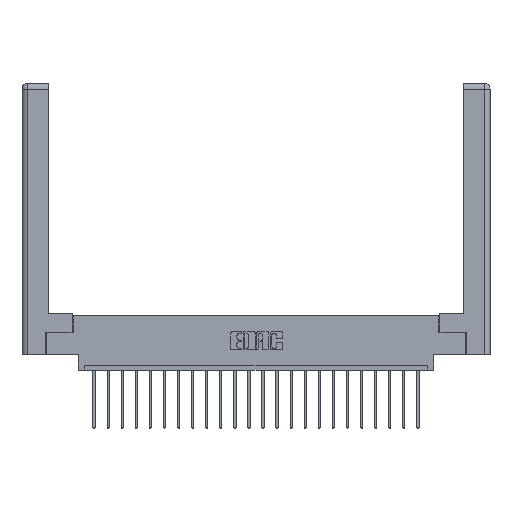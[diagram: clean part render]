
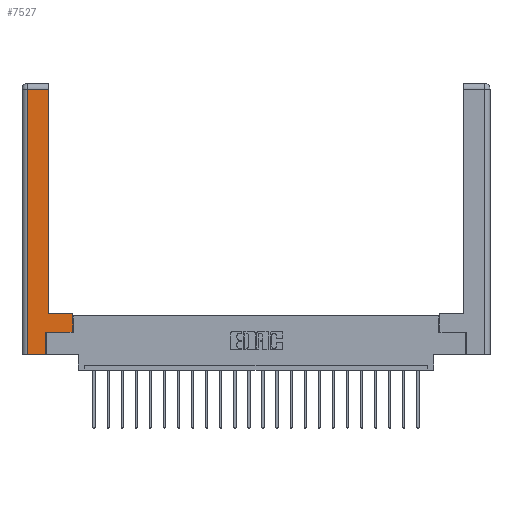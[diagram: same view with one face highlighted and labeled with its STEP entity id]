
A CAD part, top view. The second image highlights one B-rep face of the part: STEP entity #7527.
In plain terms, the highlighted planar face has unit normal (0, 0, 1).
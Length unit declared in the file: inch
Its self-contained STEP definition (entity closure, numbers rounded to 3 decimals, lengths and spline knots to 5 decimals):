
#13 = VERTEX_POINT ( 'NONE', #22347 ) ;
#789 = DIRECTION ( 'NONE',  ( 0., 0., -1. ) ) ;
#1394 = EDGE_LOOP ( 'NONE', ( #8591, #16067, #6694, #7292, #8534, #3660, #19347, #2875 ) ) ;
#1465 = VECTOR ( 'NONE', #11779, 39.37008 ) ;
#2540 = EDGE_CURVE ( 'NONE', #13, #6103, #13324, .T. ) ;
#2652 = CARTESIAN_POINT ( 'NONE',  ( 0.565, 0.45, 0. ) ) ;
#2875 = ORIENTED_EDGE ( 'NONE', *, *, #2540, .T. ) ;
#3145 = DIRECTION ( 'NONE',  ( -1., 0., 0. ) ) ;
#3184 = FACE_OUTER_BOUND ( 'NONE', #1394, .T. ) ;
#3660 = ORIENTED_EDGE ( 'NONE', *, *, #14101, .T. ) ;
#4850 = VECTOR ( 'NONE', #7792, 39.37008 ) ;
#5089 = LINE ( 'NONE', #7409, #16916 ) ;
#6103 = VERTEX_POINT ( 'NONE', #15973 ) ;
#6434 = LINE ( 'NONE', #12793, #10860 ) ;
#6504 = CARTESIAN_POINT ( 'NONE',  ( 0.265, 0., 0. ) ) ;
#6694 = ORIENTED_EDGE ( 'NONE', *, *, #9083, .T. ) ;
#6867 = VERTEX_POINT ( 'NONE', #6504 ) ;
#7292 = ORIENTED_EDGE ( 'NONE', *, *, #20407, .T. ) ;
#7409 = CARTESIAN_POINT ( 'NONE',  ( 0.265, 0.245, 0. ) ) ;
#7527 = ADVANCED_FACE ( 'NONE', ( #3184 ), #14182, .F. ) ;
#7792 = DIRECTION ( 'NONE',  ( 0., -1., 0. ) ) ;
#7862 = LINE ( 'NONE', #22399, #1465 ) ;
#8031 = EDGE_CURVE ( 'NONE', #15793, #13, #12099, .T. ) ;
#8261 = VECTOR ( 'NONE', #3145, 39.37008 ) ;
#8534 = ORIENTED_EDGE ( 'NONE', *, *, #10175, .T. ) ;
#8590 = CARTESIAN_POINT ( 'NONE',  ( 0.295, 2.94, 0. ) ) ;
#8591 = ORIENTED_EDGE ( 'NONE', *, *, #13149, .T. ) ;
#9054 = CARTESIAN_POINT ( 'NONE',  ( 0.295, 0.45, 0. ) ) ;
#9083 = EDGE_CURVE ( 'NONE', #17619, #17204, #16437, .T. ) ;
#9647 = VECTOR ( 'NONE', #16736, 39.37008 ) ;
#10175 = EDGE_CURVE ( 'NONE', #6867, #16735, #5089, .T. ) ;
#10658 = CARTESIAN_POINT ( 'NONE',  ( 0.265, 0.245, 0. ) ) ;
#10860 = VECTOR ( 'NONE', #18031, 39.37008 ) ;
#11485 = CARTESIAN_POINT ( 'NONE',  ( 0.0615, 0., 0. ) ) ;
#11603 = VERTEX_POINT ( 'NONE', #8590 ) ;
#11779 = DIRECTION ( 'NONE',  ( 1., 0., 0. ) ) ;
#12099 = LINE ( 'NONE', #2652, #17612 ) ;
#12637 = DIRECTION ( 'NONE',  ( 0., 1., 0. ) ) ;
#12793 = CARTESIAN_POINT ( 'NONE',  ( 0.295, 3., 0. ) ) ;
#13149 = EDGE_CURVE ( 'NONE', #6103, #11603, #6434, .T. ) ;
#13324 = LINE ( 'NONE', #9054, #16613 ) ;
#14101 = EDGE_CURVE ( 'NONE', #16735, #15793, #7862, .T. ) ;
#14182 = PLANE ( 'NONE',  #15507 ) ;
#14293 = CARTESIAN_POINT ( 'NONE',  ( 0.565, 0.245, 0. ) ) ;
#15154 = LINE ( 'NONE', #18975, #8261 ) ;
#15507 = AXIS2_PLACEMENT_3D ( 'NONE', #18709, #789, #16743 ) ;
#15793 = VERTEX_POINT ( 'NONE', #14293 ) ;
#15973 = CARTESIAN_POINT ( 'NONE',  ( 0.295, 0.45, 0. ) ) ;
#16034 = LINE ( 'NONE', #22375, #9647 ) ;
#16067 = ORIENTED_EDGE ( 'NONE', *, *, #21218, .T. ) ;
#16437 = LINE ( 'NONE', #11485, #4850 ) ;
#16613 = VECTOR ( 'NONE', #21283, 39.37008 ) ;
#16735 = VERTEX_POINT ( 'NONE', #10658 ) ;
#16736 = DIRECTION ( 'NONE',  ( 1., 0., 0. ) ) ;
#16743 = DIRECTION ( 'NONE',  ( -1., 0., 0. ) ) ;
#16916 = VECTOR ( 'NONE', #12637, 39.37008 ) ;
#17204 = VERTEX_POINT ( 'NONE', #22617 ) ;
#17612 = VECTOR ( 'NONE', #20827, 39.37008 ) ;
#17619 = VERTEX_POINT ( 'NONE', #22929 ) ;
#18031 = DIRECTION ( 'NONE',  ( 0., 1., 0. ) ) ;
#18709 = CARTESIAN_POINT ( 'NONE',  ( 0., 0., 0. ) ) ;
#18975 = CARTESIAN_POINT ( 'NONE',  ( 0.0615, 2.94, 0. ) ) ;
#19347 = ORIENTED_EDGE ( 'NONE', *, *, #8031, .T. ) ;
#20407 = EDGE_CURVE ( 'NONE', #17204, #6867, #16034, .T. ) ;
#20827 = DIRECTION ( 'NONE',  ( 0., 1., 0. ) ) ;
#21218 = EDGE_CURVE ( 'NONE', #11603, #17619, #15154, .T. ) ;
#21283 = DIRECTION ( 'NONE',  ( -1., 0., 0. ) ) ;
#22347 = CARTESIAN_POINT ( 'NONE',  ( 0.565, 0.45, 0. ) ) ;
#22375 = CARTESIAN_POINT ( 'NONE',  ( 0.265, 0., 0. ) ) ;
#22399 = CARTESIAN_POINT ( 'NONE',  ( 0.565, 0.245, 0. ) ) ;
#22617 = CARTESIAN_POINT ( 'NONE',  ( 0.0615, 0., 0. ) ) ;
#22929 = CARTESIAN_POINT ( 'NONE',  ( 0.0615, 2.94, 0. ) ) ;
